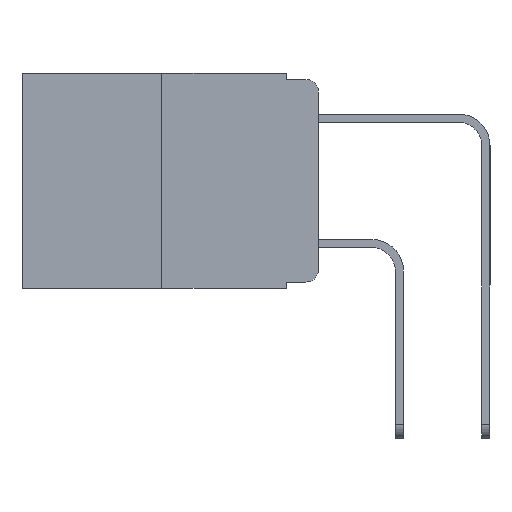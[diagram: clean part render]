
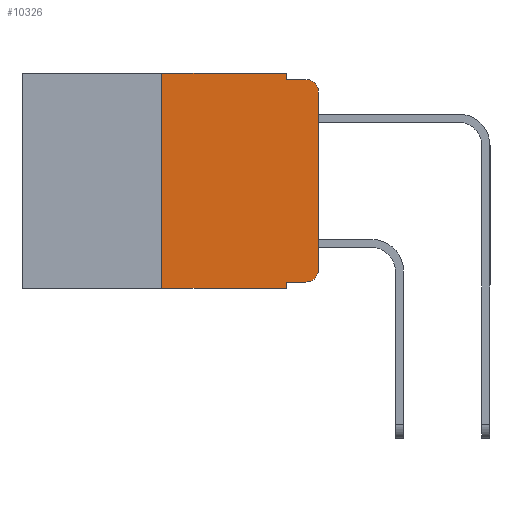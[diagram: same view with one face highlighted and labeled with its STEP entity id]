
A CAD part, left-side view. The second image highlights one B-rep face of the part: STEP entity #10326.
In plain terms, the highlighted planar face has unit normal (-1, 0, 0).
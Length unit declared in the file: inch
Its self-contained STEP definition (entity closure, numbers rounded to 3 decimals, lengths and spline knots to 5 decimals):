
#99 = LINE ( 'NONE', #2487, #18912 ) ;
#275 = EDGE_CURVE ( 'NONE', #18193, #5995, #3929, .T. ) ;
#436 = CARTESIAN_POINT ( 'NONE',  ( 0., 0., 0. ) ) ;
#747 = EDGE_CURVE ( 'NONE', #22064, #4919, #17831, .T. ) ;
#877 = AXIS2_PLACEMENT_3D ( 'NONE', #9634, #22133, #11400 ) ;
#995 = VERTEX_POINT ( 'NONE', #21060 ) ;
#1346 = DIRECTION ( 'NONE',  ( 0., 0., -1. ) ) ;
#1944 = LINE ( 'NONE', #8563, #6860 ) ;
#2039 = CARTESIAN_POINT ( 'NONE',  ( 0., 0., -0.313 ) ) ;
#2487 = CARTESIAN_POINT ( 'NONE',  ( 0., 0.473, -0.343 ) ) ;
#2574 = DIRECTION ( 'NONE',  ( 0., -1., 0. ) ) ;
#3102 = CARTESIAN_POINT ( 'NONE',  ( 0., 0.051, -0.01 ) ) ;
#3257 = VERTEX_POINT ( 'NONE', #8426 ) ;
#3644 = ORIENTED_EDGE ( 'NONE', *, *, #14902, .F. ) ;
#3929 = LINE ( 'NONE', #436, #13032 ) ;
#3939 = CARTESIAN_POINT ( 'NONE',  ( 0., 0.051, 0. ) ) ;
#4509 = VECTOR ( 'NONE', #21635, 39.37008 ) ;
#4915 = DIRECTION ( 'NONE',  ( 0., -1., 0. ) ) ;
#4919 = VERTEX_POINT ( 'NONE', #12379 ) ;
#5154 = VECTOR ( 'NONE', #17665, 39.37008 ) ;
#5459 = VECTOR ( 'NONE', #6267, 39.37008 ) ;
#5642 = ORIENTED_EDGE ( 'NONE', *, *, #275, .T. ) ;
#5995 = VERTEX_POINT ( 'NONE', #11599 ) ;
#6267 = DIRECTION ( 'NONE',  ( 0., 0., 1. ) ) ;
#6860 = VECTOR ( 'NONE', #4915, 39.37008 ) ;
#6932 = CARTESIAN_POINT ( 'NONE',  ( 0., 0.02, -0.333 ) ) ;
#7186 = LINE ( 'NONE', #3102, #16255 ) ;
#7298 = VERTEX_POINT ( 'NONE', #10104 ) ;
#8009 = DIRECTION ( 'NONE',  ( -1., 0., 0. ) ) ;
#8239 = EDGE_CURVE ( 'NONE', #4919, #995, #7186, .T. ) ;
#8426 = CARTESIAN_POINT ( 'NONE',  ( 0., 0.051, -0.343 ) ) ;
#8563 = CARTESIAN_POINT ( 'NONE',  ( 0., 0.051, -0.333 ) ) ;
#8717 = PLANE ( 'NONE',  #12753 ) ;
#8874 = EDGE_CURVE ( 'NONE', #21021, #19197, #1944, .T. ) ;
#9398 = LINE ( 'NONE', #18097, #4509 ) ;
#9634 = CARTESIAN_POINT ( 'NONE',  ( 0., 0.02, -0.313 ) ) ;
#9750 = LINE ( 'NONE', #9935, #5459 ) ;
#9935 = CARTESIAN_POINT ( 'NONE',  ( 0., 0.25, 0. ) ) ;
#9961 = CARTESIAN_POINT ( 'NONE',  ( 0., 0.25, -0.343 ) ) ;
#10028 = LINE ( 'NONE', #10396, #5154 ) ;
#10104 = CARTESIAN_POINT ( 'NONE',  ( 0., 0.25, 0. ) ) ;
#10326 = ADVANCED_FACE ( 'NONE', ( #20181 ), #8717, .F. ) ;
#10396 = CARTESIAN_POINT ( 'NONE',  ( 0., 0.473, 0. ) ) ;
#10464 = DIRECTION ( 'NONE',  ( 0., -1., 0. ) ) ;
#10502 = CARTESIAN_POINT ( 'NONE',  ( 0., 0.473, 0. ) ) ;
#11059 = ORIENTED_EDGE ( 'NONE', *, *, #18323, .T. ) ;
#11234 = CIRCLE ( 'NONE', #23141, 0.02 ) ;
#11400 = DIRECTION ( 'NONE',  ( 0., 0., -1. ) ) ;
#11599 = CARTESIAN_POINT ( 'NONE',  ( 0., 0., -0.03 ) ) ;
#12196 = CARTESIAN_POINT ( 'NONE',  ( 0., 0.051, -0.333 ) ) ;
#12197 = ORIENTED_EDGE ( 'NONE', *, *, #15110, .F. ) ;
#12286 = DIRECTION ( 'NONE',  ( 1., 0., 0. ) ) ;
#12379 = CARTESIAN_POINT ( 'NONE',  ( 0., 0.051, -0.01 ) ) ;
#12753 = AXIS2_PLACEMENT_3D ( 'NONE', #10502, #12286, #1346 ) ;
#13032 = VECTOR ( 'NONE', #16936, 39.37008 ) ;
#13620 = ORIENTED_EDGE ( 'NONE', *, *, #19551, .T. ) ;
#13828 = DIRECTION ( 'NONE',  ( 0., 0., -1. ) ) ;
#13889 = ORIENTED_EDGE ( 'NONE', *, *, #20851, .T. ) ;
#14505 = VERTEX_POINT ( 'NONE', #9961 ) ;
#14700 = ORIENTED_EDGE ( 'NONE', *, *, #16452, .F. ) ;
#14725 = VECTOR ( 'NONE', #13828, 39.37008 ) ;
#14902 = EDGE_CURVE ( 'NONE', #14505, #7298, #9750, .T. ) ;
#15110 = EDGE_CURVE ( 'NONE', #7298, #22064, #10028, .T. ) ;
#15925 = ORIENTED_EDGE ( 'NONE', *, *, #747, .F. ) ;
#16255 = VECTOR ( 'NONE', #10464, 39.37008 ) ;
#16452 = EDGE_CURVE ( 'NONE', #21021, #3257, #9398, .T. ) ;
#16936 = DIRECTION ( 'NONE',  ( 0., 0., 1. ) ) ;
#17665 = DIRECTION ( 'NONE',  ( 0., -1., 0. ) ) ;
#17831 = LINE ( 'NONE', #19527, #14725 ) ;
#18097 = CARTESIAN_POINT ( 'NONE',  ( 0., 0.051, 0. ) ) ;
#18193 = VERTEX_POINT ( 'NONE', #2039 ) ;
#18323 = EDGE_CURVE ( 'NONE', #5995, #995, #11234, .T. ) ;
#18606 = CIRCLE ( 'NONE', #877, 0.02 ) ;
#18763 = CARTESIAN_POINT ( 'NONE',  ( 0., 0.02, -0.03 ) ) ;
#18912 = VECTOR ( 'NONE', #2574, 39.37008 ) ;
#19197 = VERTEX_POINT ( 'NONE', #6932 ) ;
#19527 = CARTESIAN_POINT ( 'NONE',  ( 0., 0.051, 0. ) ) ;
#19551 = EDGE_CURVE ( 'NONE', #14505, #3257, #99, .T. ) ;
#20181 = FACE_OUTER_BOUND ( 'NONE', #22847, .T. ) ;
#20538 = DIRECTION ( 'NONE',  ( 0., 0., -1. ) ) ;
#20851 = EDGE_CURVE ( 'NONE', #19197, #18193, #18606, .T. ) ;
#21021 = VERTEX_POINT ( 'NONE', #12196 ) ;
#21060 = CARTESIAN_POINT ( 'NONE',  ( 0., 0.02, -0.01 ) ) ;
#21635 = DIRECTION ( 'NONE',  ( 0., 0., -1. ) ) ;
#22064 = VERTEX_POINT ( 'NONE', #3939 ) ;
#22133 = DIRECTION ( 'NONE',  ( -1., 0., 0. ) ) ;
#22744 = ORIENTED_EDGE ( 'NONE', *, *, #8874, .T. ) ;
#22847 = EDGE_LOOP ( 'NONE', ( #5642, #11059, #23013, #15925, #12197, #3644, #13620, #14700, #22744, #13889 ) ) ;
#23013 = ORIENTED_EDGE ( 'NONE', *, *, #8239, .F. ) ;
#23141 = AXIS2_PLACEMENT_3D ( 'NONE', #18763, #8009, #20538 ) ;
